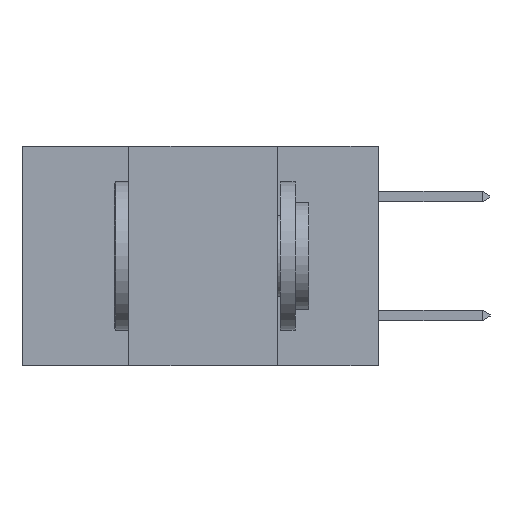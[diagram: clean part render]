
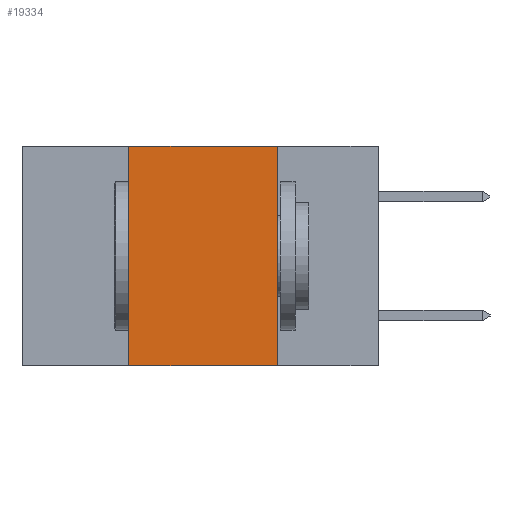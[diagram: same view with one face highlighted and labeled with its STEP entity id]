
A CAD part, left-side view. The second image highlights one B-rep face of the part: STEP entity #19334.
In plain terms, the highlighted planar face has unit normal (-1, 0, 0).
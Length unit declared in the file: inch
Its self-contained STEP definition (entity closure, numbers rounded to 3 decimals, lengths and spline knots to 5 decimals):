
#242 = LINE ( 'NONE', #7199, #12327 ) ;
#361 = CARTESIAN_POINT ( 'NONE',  ( 0., 0.6, 0. ) ) ;
#593 = VECTOR ( 'NONE', #10054, 39.37008 ) ;
#607 = VERTEX_POINT ( 'NONE', #8940 ) ;
#1034 = CARTESIAN_POINT ( 'NONE',  ( 0., 0.6, -0.37 ) ) ;
#1951 = DIRECTION ( 'NONE',  ( 0., -1., 0. ) ) ;
#2629 = AXIS2_PLACEMENT_3D ( 'NONE', #17037, #18581, #9258 ) ;
#2654 = LINE ( 'NONE', #361, #14663 ) ;
#4274 = LINE ( 'NONE', #8486, #593 ) ;
#5699 = ORIENTED_EDGE ( 'NONE', *, *, #15287, .T. ) ;
#5843 = CARTESIAN_POINT ( 'NONE',  ( 0., 0.42, 0. ) ) ;
#6471 = EDGE_CURVE ( 'NONE', #7762, #18630, #242, .T. ) ;
#6515 = FACE_OUTER_BOUND ( 'NONE', #12193, .T. ) ;
#7199 = CARTESIAN_POINT ( 'NONE',  ( 0., 0.42, -0.37 ) ) ;
#7595 = CARTESIAN_POINT ( 'NONE',  ( 0., 0.17, -0.37 ) ) ;
#7762 = VERTEX_POINT ( 'NONE', #18265 ) ;
#8189 = EDGE_CURVE ( 'NONE', #18630, #607, #2654, .T. ) ;
#8486 = CARTESIAN_POINT ( 'NONE',  ( 0., 0.17, -0.37 ) ) ;
#8940 = CARTESIAN_POINT ( 'NONE',  ( 0., 0.17, 0. ) ) ;
#9258 = DIRECTION ( 'NONE',  ( 0., 0., -1. ) ) ;
#10054 = DIRECTION ( 'NONE',  ( 0., 0., -1. ) ) ;
#10469 = DIRECTION ( 'NONE',  ( 0., -1., 0. ) ) ;
#11387 = LINE ( 'NONE', #1034, #19143 ) ;
#12193 = EDGE_LOOP ( 'NONE', ( #16435, #14741, #13086, #5699 ) ) ;
#12327 = VECTOR ( 'NONE', #16556, 39.37008 ) ;
#13086 = ORIENTED_EDGE ( 'NONE', *, *, #6471, .F. ) ;
#14663 = VECTOR ( 'NONE', #1951, 39.37008 ) ;
#14741 = ORIENTED_EDGE ( 'NONE', *, *, #8189, .F. ) ;
#15287 = EDGE_CURVE ( 'NONE', #7762, #19949, #11387, .T. ) ;
#15488 = PLANE ( 'NONE',  #2629 ) ;
#16435 = ORIENTED_EDGE ( 'NONE', *, *, #19688, .F. ) ;
#16556 = DIRECTION ( 'NONE',  ( 0., 0., 1. ) ) ;
#17037 = CARTESIAN_POINT ( 'NONE',  ( 0., 0.6, 0. ) ) ;
#18265 = CARTESIAN_POINT ( 'NONE',  ( 0., 0.42, -0.37 ) ) ;
#18581 = DIRECTION ( 'NONE',  ( 1., 0., 0. ) ) ;
#18630 = VERTEX_POINT ( 'NONE', #5843 ) ;
#19143 = VECTOR ( 'NONE', #10469, 39.37008 ) ;
#19334 = ADVANCED_FACE ( 'NONE', ( #6515 ), #15488, .F. ) ;
#19688 = EDGE_CURVE ( 'NONE', #607, #19949, #4274, .T. ) ;
#19949 = VERTEX_POINT ( 'NONE', #7595 ) ;
